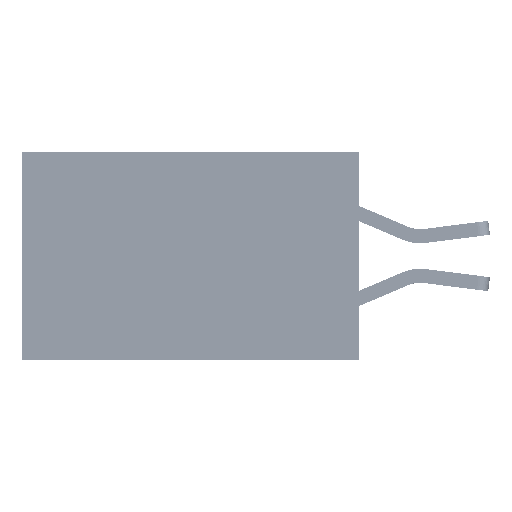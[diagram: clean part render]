
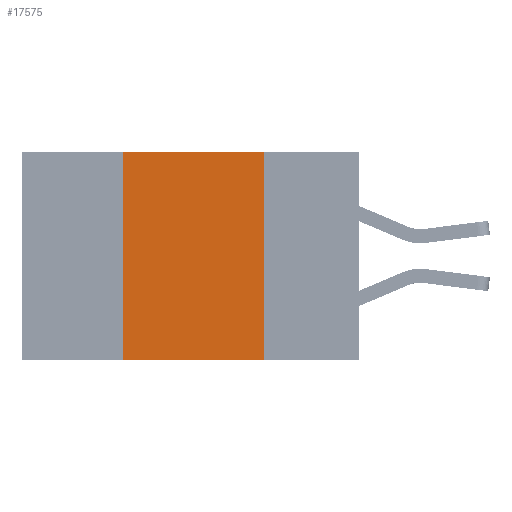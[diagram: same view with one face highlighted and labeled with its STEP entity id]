
A CAD part, left-side view. The second image highlights one B-rep face of the part: STEP entity #17575.
In plain terms, the highlighted planar face has unit normal (-1, 0, 0).
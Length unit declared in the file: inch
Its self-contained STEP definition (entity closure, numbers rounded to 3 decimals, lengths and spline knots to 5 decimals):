
#937 = CARTESIAN_POINT ( 'NONE',  ( 0., 0.17, 0. ) ) ;
#957 = VECTOR ( 'NONE', #3781, 39.37008 ) ;
#1002 = ORIENTED_EDGE ( 'NONE', *, *, #2164, .F. ) ;
#1946 = DIRECTION ( 'NONE',  ( 1., 0., 0. ) ) ;
#2103 = CARTESIAN_POINT ( 'NONE',  ( 0., 0.42, 0. ) ) ;
#2164 = EDGE_CURVE ( 'NONE', #22715, #9164, #39074, .T. ) ;
#3781 = DIRECTION ( 'NONE',  ( 0., 0., -1. ) ) ;
#3869 = VERTEX_POINT ( 'NONE', #34913 ) ;
#8147 = AXIS2_PLACEMENT_3D ( 'NONE', #21760, #1946, #28282 ) ;
#8210 = CARTESIAN_POINT ( 'NONE',  ( 0., 0.42, -0.37 ) ) ;
#9164 = VERTEX_POINT ( 'NONE', #24216 ) ;
#9589 = EDGE_CURVE ( 'NONE', #9164, #24683, #13069, .T. ) ;
#12348 = CARTESIAN_POINT ( 'NONE',  ( 0., 0.6, -0.37 ) ) ;
#12478 = ORIENTED_EDGE ( 'NONE', *, *, #9589, .F. ) ;
#13069 = LINE ( 'NONE', #26345, #23681 ) ;
#17575 = ADVANCED_FACE ( 'NONE', ( #38272 ), #27860, .F. ) ;
#19755 = VECTOR ( 'NONE', #41908, 39.37008 ) ;
#21760 = CARTESIAN_POINT ( 'NONE',  ( 0., 0.6, 0. ) ) ;
#22321 = ORIENTED_EDGE ( 'NONE', *, *, #34231, .T. ) ;
#22502 = EDGE_LOOP ( 'NONE', ( #28385, #12478, #1002, #22321 ) ) ;
#22715 = VERTEX_POINT ( 'NONE', #8210 ) ;
#23562 = EDGE_CURVE ( 'NONE', #24683, #3869, #24452, .T. ) ;
#23681 = VECTOR ( 'NONE', #39602, 39.37008 ) ;
#24216 = CARTESIAN_POINT ( 'NONE',  ( 0., 0.42, 0. ) ) ;
#24452 = LINE ( 'NONE', #937, #957 ) ;
#24683 = VERTEX_POINT ( 'NONE', #32406 ) ;
#26345 = CARTESIAN_POINT ( 'NONE',  ( 0., 0.6, 0. ) ) ;
#27860 = PLANE ( 'NONE',  #8147 ) ;
#28282 = DIRECTION ( 'NONE',  ( 0., 0., -1. ) ) ;
#28385 = ORIENTED_EDGE ( 'NONE', *, *, #23562, .F. ) ;
#32150 = VECTOR ( 'NONE', #41508, 39.37008 ) ;
#32406 = CARTESIAN_POINT ( 'NONE',  ( 0., 0.17, 0. ) ) ;
#34231 = EDGE_CURVE ( 'NONE', #22715, #3869, #41721, .T. ) ;
#34913 = CARTESIAN_POINT ( 'NONE',  ( 0., 0.17, -0.37 ) ) ;
#38272 = FACE_OUTER_BOUND ( 'NONE', #22502, .T. ) ;
#39074 = LINE ( 'NONE', #2103, #19755 ) ;
#39602 = DIRECTION ( 'NONE',  ( 0., -1., 0. ) ) ;
#41508 = DIRECTION ( 'NONE',  ( 0., -1., 0. ) ) ;
#41721 = LINE ( 'NONE', #12348, #32150 ) ;
#41908 = DIRECTION ( 'NONE',  ( 0., 0., 1. ) ) ;
